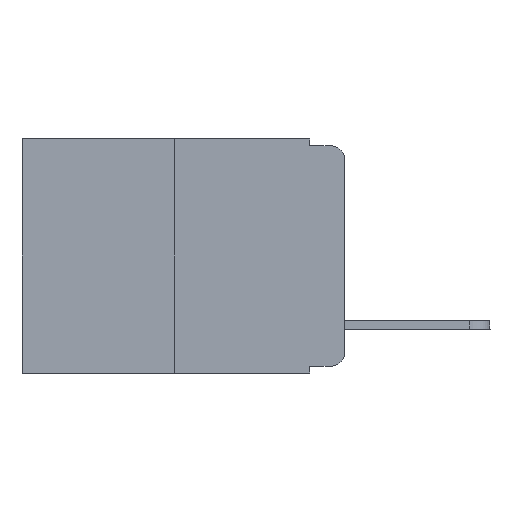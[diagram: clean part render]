
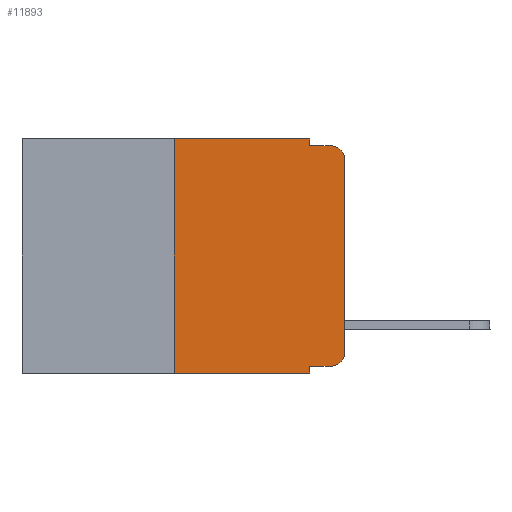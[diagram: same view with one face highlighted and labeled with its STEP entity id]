
A CAD part, left-side view. The second image highlights one B-rep face of the part: STEP entity #11893.
In plain terms, the highlighted planar face has unit normal (-1, 0, 0).
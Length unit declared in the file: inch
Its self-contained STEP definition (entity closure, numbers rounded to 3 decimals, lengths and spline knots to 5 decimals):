
#14 = ORIENTED_EDGE ( 'NONE', *, *, #8400, .F. ) ;
#45 = VERTEX_POINT ( 'NONE', #15419 ) ;
#69 = CARTESIAN_POINT ( 'NONE',  ( 0., 0.02, -0.03 ) ) ;
#444 = VECTOR ( 'NONE', #8314, 39.37008 ) ;
#534 = VECTOR ( 'NONE', #14884, 39.37008 ) ;
#593 = CARTESIAN_POINT ( 'NONE',  ( 0., 0., -0.03 ) ) ;
#1315 = VECTOR ( 'NONE', #16153, 39.37008 ) ;
#1347 = AXIS2_PLACEMENT_3D ( 'NONE', #15365, #4089, #4178 ) ;
#1956 = EDGE_CURVE ( 'NONE', #9901, #45, #13934, .T. ) ;
#2209 = CARTESIAN_POINT ( 'NONE',  ( 0., 0.473, -0.343 ) ) ;
#3206 = DIRECTION ( 'NONE',  ( 0., 0., -1. ) ) ;
#3356 = CARTESIAN_POINT ( 'NONE',  ( 0., 0.473, 0. ) ) ;
#3415 = DIRECTION ( 'NONE',  ( 0., -1., 0. ) ) ;
#3504 = CARTESIAN_POINT ( 'NONE',  ( 0., 0.051, -0.01 ) ) ;
#3650 = CARTESIAN_POINT ( 'NONE',  ( 0., 0.25, 0. ) ) ;
#3671 = VERTEX_POINT ( 'NONE', #10431 ) ;
#3694 = CARTESIAN_POINT ( 'NONE',  ( 0., 0.051, -0.343 ) ) ;
#3880 = EDGE_CURVE ( 'NONE', #10085, #6142, #13442, .T. ) ;
#3938 = EDGE_CURVE ( 'NONE', #3671, #9861, #6161, .T. ) ;
#4089 = DIRECTION ( 'NONE',  ( -1., 0., 0. ) ) ;
#4106 = LINE ( 'NONE', #15213, #8403 ) ;
#4178 = DIRECTION ( 'NONE',  ( 0., 0., -1. ) ) ;
#4386 = CARTESIAN_POINT ( 'NONE',  ( 0., 0.051, -0.333 ) ) ;
#5100 = DIRECTION ( 'NONE',  ( -1., 0., 0. ) ) ;
#5119 = DIRECTION ( 'NONE',  ( 0., 0., -1. ) ) ;
#5294 = AXIS2_PLACEMENT_3D ( 'NONE', #3356, #7017, #3206 ) ;
#5433 = VERTEX_POINT ( 'NONE', #4386 ) ;
#5488 = CARTESIAN_POINT ( 'NONE',  ( 0., 0.02, -0.01 ) ) ;
#5764 = EDGE_CURVE ( 'NONE', #5433, #9901, #9956, .T. ) ;
#5878 = ORIENTED_EDGE ( 'NONE', *, *, #12114, .F. ) ;
#6021 = PLANE ( 'NONE',  #5294 ) ;
#6142 = VERTEX_POINT ( 'NONE', #10015 ) ;
#6161 = LINE ( 'NONE', #3504, #6279 ) ;
#6279 = VECTOR ( 'NONE', #3415, 39.37008 ) ;
#6607 = EDGE_LOOP ( 'NONE', ( #11133, #10933, #12779, #14, #12320, #11026, #15527, #5878, #13246, #14498 ) ) ;
#6826 = VECTOR ( 'NONE', #10551, 39.37008 ) ;
#7017 = DIRECTION ( 'NONE',  ( 1., 0., 0. ) ) ;
#7057 = EDGE_CURVE ( 'NONE', #12722, #9861, #15677, .T. ) ;
#7259 = EDGE_CURVE ( 'NONE', #13363, #15200, #11005, .T. ) ;
#7626 = CARTESIAN_POINT ( 'NONE',  ( 0., 0.25, 0. ) ) ;
#8314 = DIRECTION ( 'NONE',  ( 0., -1., 0. ) ) ;
#8400 = EDGE_CURVE ( 'NONE', #6142, #3671, #4106, .T. ) ;
#8403 = VECTOR ( 'NONE', #5119, 39.37008 ) ;
#8593 = EDGE_CURVE ( 'NONE', #45, #12722, #13227, .T. ) ;
#8740 = CARTESIAN_POINT ( 'NONE',  ( 0., 0.051, -0.333 ) ) ;
#8747 = CARTESIAN_POINT ( 'NONE',  ( 0., 0.25, -0.343 ) ) ;
#8901 = DIRECTION ( 'NONE',  ( 0., -1., 0. ) ) ;
#9146 = EDGE_CURVE ( 'NONE', #13363, #10085, #12605, .T. ) ;
#9861 = VERTEX_POINT ( 'NONE', #5488 ) ;
#9901 = VERTEX_POINT ( 'NONE', #13424 ) ;
#9956 = LINE ( 'NONE', #8740, #16176 ) ;
#9958 = LINE ( 'NONE', #16263, #534 ) ;
#10015 = CARTESIAN_POINT ( 'NONE',  ( 0., 0.051, 0. ) ) ;
#10085 = VERTEX_POINT ( 'NONE', #7626 ) ;
#10117 = DIRECTION ( 'NONE',  ( 0., 0., -1. ) ) ;
#10431 = CARTESIAN_POINT ( 'NONE',  ( 0., 0.051, -0.01 ) ) ;
#10551 = DIRECTION ( 'NONE',  ( 0., 0., 1. ) ) ;
#10933 = ORIENTED_EDGE ( 'NONE', *, *, #7057, .T. ) ;
#11005 = LINE ( 'NONE', #2209, #444 ) ;
#11026 = ORIENTED_EDGE ( 'NONE', *, *, #9146, .F. ) ;
#11133 = ORIENTED_EDGE ( 'NONE', *, *, #8593, .T. ) ;
#11893 = ADVANCED_FACE ( 'NONE', ( #14635 ), #6021, .F. ) ;
#12114 = EDGE_CURVE ( 'NONE', #5433, #15200, #9958, .T. ) ;
#12320 = ORIENTED_EDGE ( 'NONE', *, *, #3880, .F. ) ;
#12605 = LINE ( 'NONE', #3650, #1315 ) ;
#12722 = VERTEX_POINT ( 'NONE', #593 ) ;
#12779 = ORIENTED_EDGE ( 'NONE', *, *, #3938, .F. ) ;
#13145 = CARTESIAN_POINT ( 'NONE',  ( 0., 0., 0. ) ) ;
#13227 = LINE ( 'NONE', #13145, #6826 ) ;
#13246 = ORIENTED_EDGE ( 'NONE', *, *, #5764, .T. ) ;
#13339 = VECTOR ( 'NONE', #13777, 39.37008 ) ;
#13363 = VERTEX_POINT ( 'NONE', #8747 ) ;
#13424 = CARTESIAN_POINT ( 'NONE',  ( 0., 0.02, -0.333 ) ) ;
#13442 = LINE ( 'NONE', #13608, #13339 ) ;
#13608 = CARTESIAN_POINT ( 'NONE',  ( 0., 0.473, 0. ) ) ;
#13777 = DIRECTION ( 'NONE',  ( 0., -1., 0. ) ) ;
#13934 = CIRCLE ( 'NONE', #1347, 0.02 ) ;
#14498 = ORIENTED_EDGE ( 'NONE', *, *, #1956, .T. ) ;
#14635 = FACE_OUTER_BOUND ( 'NONE', #6607, .T. ) ;
#14884 = DIRECTION ( 'NONE',  ( 0., 0., -1. ) ) ;
#14915 = AXIS2_PLACEMENT_3D ( 'NONE', #69, #5100, #10117 ) ;
#15200 = VERTEX_POINT ( 'NONE', #3694 ) ;
#15213 = CARTESIAN_POINT ( 'NONE',  ( 0., 0.051, 0. ) ) ;
#15365 = CARTESIAN_POINT ( 'NONE',  ( 0., 0.02, -0.313 ) ) ;
#15419 = CARTESIAN_POINT ( 'NONE',  ( 0., 0., -0.313 ) ) ;
#15527 = ORIENTED_EDGE ( 'NONE', *, *, #7259, .T. ) ;
#15677 = CIRCLE ( 'NONE', #14915, 0.02 ) ;
#16153 = DIRECTION ( 'NONE',  ( 0., 0., 1. ) ) ;
#16176 = VECTOR ( 'NONE', #8901, 39.37008 ) ;
#16263 = CARTESIAN_POINT ( 'NONE',  ( 0., 0.051, 0. ) ) ;
